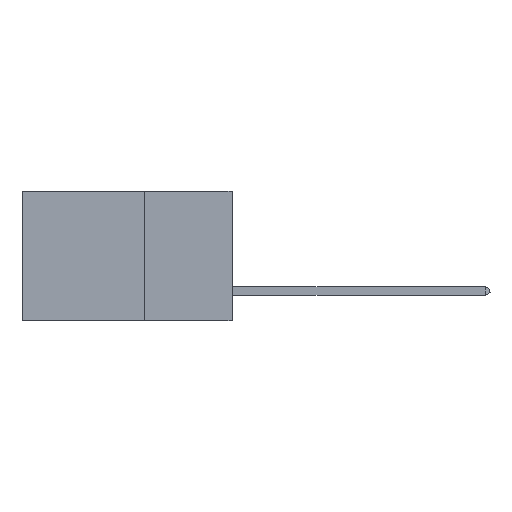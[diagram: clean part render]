
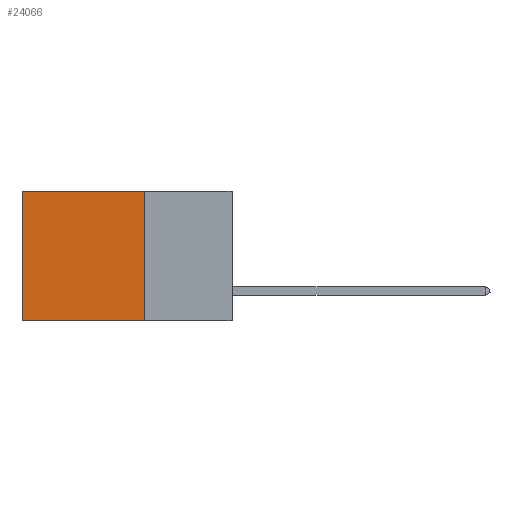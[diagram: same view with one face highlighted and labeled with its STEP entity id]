
A CAD part, left-side view. The second image highlights one B-rep face of the part: STEP entity #24066.
In plain terms, the highlighted planar face has unit normal (-1, 0, 0).
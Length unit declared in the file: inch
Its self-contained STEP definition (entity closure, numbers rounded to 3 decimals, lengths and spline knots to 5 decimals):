
#81 = LINE ( 'NONE', #30623, #3140 ) ;
#1749 = VECTOR ( 'NONE', #17736, 39.37008 ) ;
#1849 = FACE_OUTER_BOUND ( 'NONE', #4035, .T. ) ;
#2167 = CARTESIAN_POINT ( 'NONE',  ( 0.2875, 0.25, 0. ) ) ;
#2410 = EDGE_CURVE ( 'NONE', #5612, #11171, #9231, .T. ) ;
#2461 = CARTESIAN_POINT ( 'NONE',  ( 0.2875, 0.25, 0. ) ) ;
#3140 = VECTOR ( 'NONE', #28480, 39.37008 ) ;
#4035 = EDGE_LOOP ( 'NONE', ( #4376, #8321, #18084, #11051 ) ) ;
#4376 = ORIENTED_EDGE ( 'NONE', *, *, #6045, .T. ) ;
#4388 = DIRECTION ( 'NONE',  ( 0., 0., -1. ) ) ;
#5612 = VERTEX_POINT ( 'NONE', #18125 ) ;
#5687 = VERTEX_POINT ( 'NONE', #17901 ) ;
#6045 = EDGE_CURVE ( 'NONE', #8587, #5687, #13144, .T. ) ;
#6524 = CARTESIAN_POINT ( 'NONE',  ( 0.2875, 0.25, 0. ) ) ;
#7402 = EDGE_CURVE ( 'NONE', #11171, #5687, #81, .T. ) ;
#7737 = LINE ( 'NONE', #2167, #18435 ) ;
#8321 = ORIENTED_EDGE ( 'NONE', *, *, #7402, .F. ) ;
#8587 = VERTEX_POINT ( 'NONE', #17363 ) ;
#9231 = LINE ( 'NONE', #6524, #25992 ) ;
#11051 = ORIENTED_EDGE ( 'NONE', *, *, #26940, .T. ) ;
#11171 = VERTEX_POINT ( 'NONE', #24909 ) ;
#13144 = LINE ( 'NONE', #25371, #1749 ) ;
#17363 = CARTESIAN_POINT ( 'NONE',  ( 0.2875, 0.6, 0. ) ) ;
#17736 = DIRECTION ( 'NONE',  ( 0., 0., -1. ) ) ;
#17901 = CARTESIAN_POINT ( 'NONE',  ( 0.2875, 0.6, -0.37 ) ) ;
#18084 = ORIENTED_EDGE ( 'NONE', *, *, #2410, .F. ) ;
#18125 = CARTESIAN_POINT ( 'NONE',  ( 0.2875, 0.25, 0. ) ) ;
#18435 = VECTOR ( 'NONE', #24417, 39.37008 ) ;
#21850 = DIRECTION ( 'NONE',  ( 1., 0., 0. ) ) ;
#24066 = ADVANCED_FACE ( 'NONE', ( #1849 ), #26702, .F. ) ;
#24417 = DIRECTION ( 'NONE',  ( 0., 1., 0. ) ) ;
#24425 = DIRECTION ( 'NONE',  ( 0., 0., -1. ) ) ;
#24909 = CARTESIAN_POINT ( 'NONE',  ( 0.2875, 0.25, -0.37 ) ) ;
#25371 = CARTESIAN_POINT ( 'NONE',  ( 0.2875, 0.6, 0. ) ) ;
#25992 = VECTOR ( 'NONE', #4388, 39.37008 ) ;
#26702 = PLANE ( 'NONE',  #28148 ) ;
#26940 = EDGE_CURVE ( 'NONE', #5612, #8587, #7737, .T. ) ;
#28148 = AXIS2_PLACEMENT_3D ( 'NONE', #2461, #21850, #24425 ) ;
#28480 = DIRECTION ( 'NONE',  ( 0., 1., 0. ) ) ;
#30623 = CARTESIAN_POINT ( 'NONE',  ( 0.2875, 0.25, -0.37 ) ) ;
